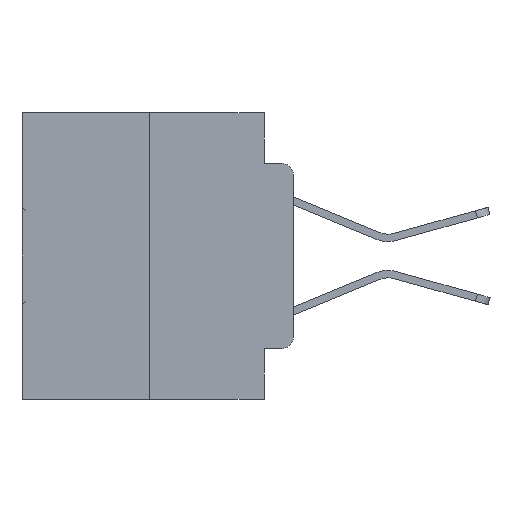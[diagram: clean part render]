
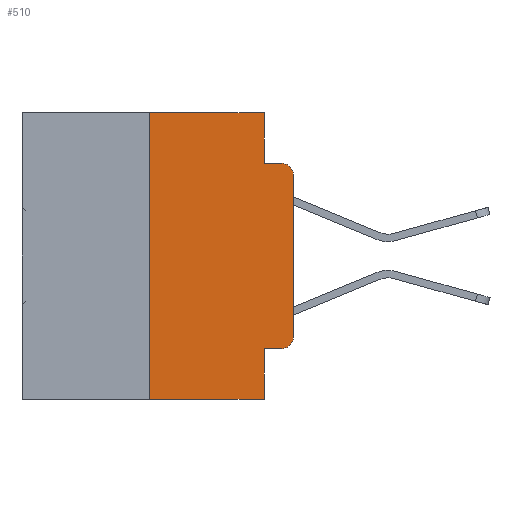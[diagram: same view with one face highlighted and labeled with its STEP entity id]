
A CAD part, left-side view. The second image highlights one B-rep face of the part: STEP entity #510.
In plain terms, the highlighted planar face has unit normal (-1, 0, 0).
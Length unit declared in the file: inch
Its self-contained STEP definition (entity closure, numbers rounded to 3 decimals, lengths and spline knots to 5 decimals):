
#271 = CIRCLE ( 'NONE', #1080, 0.02 ) ;
#510 = ADVANCED_FACE ( 'NONE', ( #1778 ), #19373, .F. ) ;
#666 = CIRCLE ( 'NONE', #14646, 0.02 ) ;
#741 = LINE ( 'NONE', #27457, #27066 ) ;
#1065 = VECTOR ( 'NONE', #30351, 39.37008 ) ;
#1080 = AXIS2_PLACEMENT_3D ( 'NONE', #32884, #16859, #32647 ) ;
#1521 = DIRECTION ( 'NONE',  ( 0., 0., 1. ) ) ;
#1681 = CARTESIAN_POINT ( 'NONE',  ( 0., 0.02, -0.0885 ) ) ;
#1778 = FACE_OUTER_BOUND ( 'NONE', #6529, .T. ) ;
#2066 = CARTESIAN_POINT ( 'NONE',  ( 0., 0.051, -0.0885 ) ) ;
#2180 = CARTESIAN_POINT ( 'NONE',  ( 0., 0.051, -0.0885 ) ) ;
#2451 = CARTESIAN_POINT ( 'NONE',  ( 0., 0.051, 0. ) ) ;
#2904 = DIRECTION ( 'NONE',  ( 0., 0., -1. ) ) ;
#3469 = EDGE_CURVE ( 'NONE', #18228, #5704, #741, .T. ) ;
#3721 = DIRECTION ( 'NONE',  ( 0., 0., -1. ) ) ;
#4442 = VERTEX_POINT ( 'NONE', #10546 ) ;
#5391 = LINE ( 'NONE', #17363, #25566 ) ;
#5704 = VERTEX_POINT ( 'NONE', #20117 ) ;
#5758 = CARTESIAN_POINT ( 'NONE',  ( 0., 0.25, -0.5 ) ) ;
#5872 = CARTESIAN_POINT ( 'NONE',  ( 0., 0.051, 0. ) ) ;
#6529 = EDGE_LOOP ( 'NONE', ( #27667, #10120, #25523, #14085, #27236, #20152, #25046, #28109, #12834, #11338 ) ) ;
#9151 = DIRECTION ( 'NONE',  ( 0., -1., 0. ) ) ;
#9250 = EDGE_CURVE ( 'NONE', #19291, #20114, #271, .T. ) ;
#9638 = EDGE_CURVE ( 'NONE', #18228, #20462, #31527, .T. ) ;
#9841 = CARTESIAN_POINT ( 'NONE',  ( 0., 0., -0.1085 ) ) ;
#10120 = ORIENTED_EDGE ( 'NONE', *, *, #9250, .T. ) ;
#10191 = EDGE_CURVE ( 'NONE', #31116, #21441, #30228, .T. ) ;
#10546 = CARTESIAN_POINT ( 'NONE',  ( 0., 0.051, -0.4115 ) ) ;
#10756 = LINE ( 'NONE', #2180, #16940 ) ;
#11338 = ORIENTED_EDGE ( 'NONE', *, *, #16963, .T. ) ;
#11812 = VECTOR ( 'NONE', #22910, 39.37008 ) ;
#12165 = CARTESIAN_POINT ( 'NONE',  ( 0., 0.051, -0.4115 ) ) ;
#12834 = ORIENTED_EDGE ( 'NONE', *, *, #16692, .T. ) ;
#12940 = VECTOR ( 'NONE', #2904, 39.37008 ) ;
#14085 = ORIENTED_EDGE ( 'NONE', *, *, #10191, .F. ) ;
#14646 = AXIS2_PLACEMENT_3D ( 'NONE', #15824, #15918, #26531 ) ;
#15824 = CARTESIAN_POINT ( 'NONE',  ( 0., 0.02, -0.3915 ) ) ;
#15918 = DIRECTION ( 'NONE',  ( -1., 0., 0. ) ) ;
#16692 = EDGE_CURVE ( 'NONE', #4442, #26734, #20066, .T. ) ;
#16859 = DIRECTION ( 'NONE',  ( -1., 0., 0. ) ) ;
#16940 = VECTOR ( 'NONE', #23128, 39.37008 ) ;
#16963 = EDGE_CURVE ( 'NONE', #26734, #18274, #666, .T. ) ;
#17255 = CARTESIAN_POINT ( 'NONE',  ( 0., 0.25, 0. ) ) ;
#17363 = CARTESIAN_POINT ( 'NONE',  ( 0., 0.473, 0. ) ) ;
#18228 = VERTEX_POINT ( 'NONE', #5758 ) ;
#18274 = VERTEX_POINT ( 'NONE', #32078 ) ;
#19291 = VERTEX_POINT ( 'NONE', #9841 ) ;
#19373 = PLANE ( 'NONE',  #23851 ) ;
#20066 = LINE ( 'NONE', #12165, #11812 ) ;
#20114 = VERTEX_POINT ( 'NONE', #1681 ) ;
#20117 = CARTESIAN_POINT ( 'NONE',  ( 0., 0.051, -0.5 ) ) ;
#20152 = ORIENTED_EDGE ( 'NONE', *, *, #9638, .F. ) ;
#20462 = VERTEX_POINT ( 'NONE', #21245 ) ;
#21049 = CARTESIAN_POINT ( 'NONE',  ( 0., 0.051, 0. ) ) ;
#21245 = CARTESIAN_POINT ( 'NONE',  ( 0., 0.25, 0. ) ) ;
#21441 = VERTEX_POINT ( 'NONE', #2066 ) ;
#21486 = EDGE_CURVE ( 'NONE', #21441, #20114, #10756, .T. ) ;
#22672 = EDGE_CURVE ( 'NONE', #20462, #31116, #5391, .T. ) ;
#22910 = DIRECTION ( 'NONE',  ( 0., -1., 0. ) ) ;
#23128 = DIRECTION ( 'NONE',  ( 0., -1., 0. ) ) ;
#23851 = AXIS2_PLACEMENT_3D ( 'NONE', #27190, #30055, #3721 ) ;
#25046 = ORIENTED_EDGE ( 'NONE', *, *, #3469, .T. ) ;
#25203 = DIRECTION ( 'NONE',  ( 0., -1., 0. ) ) ;
#25523 = ORIENTED_EDGE ( 'NONE', *, *, #21486, .F. ) ;
#25566 = VECTOR ( 'NONE', #25203, 39.37008 ) ;
#26531 = DIRECTION ( 'NONE',  ( 0., 0., -1. ) ) ;
#26734 = VERTEX_POINT ( 'NONE', #27556 ) ;
#26922 = VECTOR ( 'NONE', #32816, 39.37008 ) ;
#27066 = VECTOR ( 'NONE', #9151, 39.37008 ) ;
#27190 = CARTESIAN_POINT ( 'NONE',  ( 0., 0.473, 0. ) ) ;
#27236 = ORIENTED_EDGE ( 'NONE', *, *, #22672, .F. ) ;
#27457 = CARTESIAN_POINT ( 'NONE',  ( 0., 0.473, -0.5 ) ) ;
#27556 = CARTESIAN_POINT ( 'NONE',  ( 0., 0.02, -0.4115 ) ) ;
#27667 = ORIENTED_EDGE ( 'NONE', *, *, #28118, .T. ) ;
#28109 = ORIENTED_EDGE ( 'NONE', *, *, #29852, .F. ) ;
#28118 = EDGE_CURVE ( 'NONE', #18274, #19291, #30290, .T. ) ;
#29852 = EDGE_CURVE ( 'NONE', #4442, #5704, #31038, .T. ) ;
#30055 = DIRECTION ( 'NONE',  ( 1., 0., 0. ) ) ;
#30228 = LINE ( 'NONE', #2451, #26922 ) ;
#30290 = LINE ( 'NONE', #33374, #1065 ) ;
#30351 = DIRECTION ( 'NONE',  ( 0., 0., 1. ) ) ;
#31038 = LINE ( 'NONE', #5872, #12940 ) ;
#31116 = VERTEX_POINT ( 'NONE', #21049 ) ;
#31527 = LINE ( 'NONE', #17255, #33588 ) ;
#32078 = CARTESIAN_POINT ( 'NONE',  ( 0., 0., -0.3915 ) ) ;
#32647 = DIRECTION ( 'NONE',  ( 0., 0., -1. ) ) ;
#32816 = DIRECTION ( 'NONE',  ( 0., 0., -1. ) ) ;
#32884 = CARTESIAN_POINT ( 'NONE',  ( 0., 0.02, -0.1085 ) ) ;
#33374 = CARTESIAN_POINT ( 'NONE',  ( 0., 0., 0. ) ) ;
#33588 = VECTOR ( 'NONE', #1521, 39.37008 ) ;
